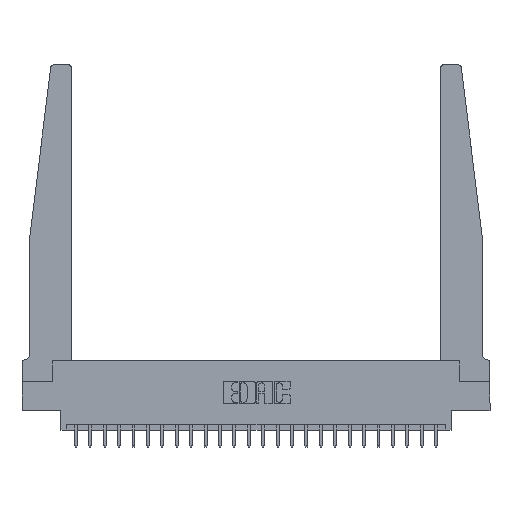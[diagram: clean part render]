
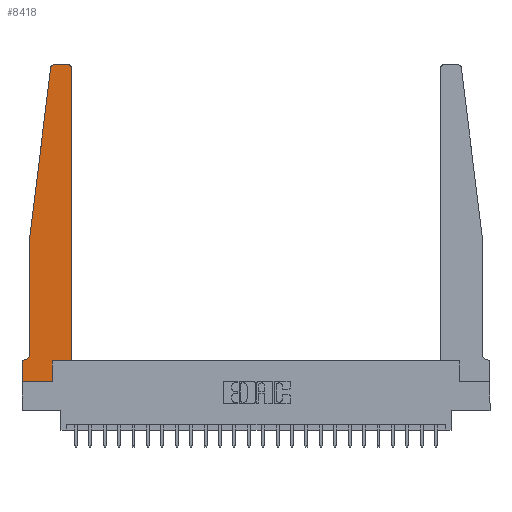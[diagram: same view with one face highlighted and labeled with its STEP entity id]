
A CAD part, top view. The second image highlights one B-rep face of the part: STEP entity #8418.
In plain terms, the highlighted planar face has unit normal (0, 0, 1).
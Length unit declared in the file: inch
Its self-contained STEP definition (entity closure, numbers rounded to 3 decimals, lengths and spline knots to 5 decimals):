
#93 = CARTESIAN_POINT ( 'NONE',  ( 0.425, 0.18, 0.37 ) ) ;
#148 = EDGE_CURVE ( 'NONE', #23735, #19029, #3038, .T. ) ;
#575 = EDGE_CURVE ( 'NONE', #8335, #3138, #4792, .T. ) ;
#618 = ORIENTED_EDGE ( 'NONE', *, *, #18903, .T. ) ;
#752 = EDGE_CURVE ( 'NONE', #6544, #5603, #20472, .T. ) ;
#990 = AXIS2_PLACEMENT_3D ( 'NONE', #11127, #23909, #12964 ) ;
#1376 = EDGE_CURVE ( 'NONE', #8189, #11717, #5085, .T. ) ;
#1635 = ORIENTED_EDGE ( 'NONE', *, *, #6350, .T. ) ;
#2336 = EDGE_CURVE ( 'NONE', #5603, #23596, #15535, .T. ) ;
#2515 = DIRECTION ( 'NONE',  ( -1., 0., 0. ) ) ;
#2861 = AXIS2_PLACEMENT_3D ( 'NONE', #17002, #5889, #18854 ) ;
#2961 = DIRECTION ( 'NONE',  ( 0., 0., 1. ) ) ;
#2983 = ORIENTED_EDGE ( 'NONE', *, *, #148, .T. ) ;
#3033 = CARTESIAN_POINT ( 'NONE',  ( 0., 0., 0.37 ) ) ;
#3038 = LINE ( 'NONE', #3033, #17319 ) ;
#3138 = VERTEX_POINT ( 'NONE', #21702 ) ;
#3180 = LINE ( 'NONE', #12296, #22329 ) ;
#3319 = ORIENTED_EDGE ( 'NONE', *, *, #752, .T. ) ;
#3325 = CARTESIAN_POINT ( 'NONE',  ( 0.2605, 0.18, 0.37 ) ) ;
#3901 = LINE ( 'NONE', #16484, #13267 ) ;
#3904 = ORIENTED_EDGE ( 'NONE', *, *, #1376, .T. ) ;
#4440 = CARTESIAN_POINT ( 'NONE',  ( 0.065, 1.25, 0.37 ) ) ;
#4792 = LINE ( 'NONE', #11908, #9237 ) ;
#5085 = LINE ( 'NONE', #21316, #9513 ) ;
#5603 = VERTEX_POINT ( 'NONE', #13830 ) ;
#5697 = VECTOR ( 'NONE', #23321, 39.37008 ) ;
#5717 = VECTOR ( 'NONE', #20847, 39.37008 ) ;
#5889 = DIRECTION ( 'NONE',  ( 0., 0., 1. ) ) ;
#6098 = FACE_OUTER_BOUND ( 'NONE', #22057, .T. ) ;
#6304 = LINE ( 'NONE', #13454, #5717 ) ;
#6350 = EDGE_CURVE ( 'NONE', #23596, #22242, #3180, .T. ) ;
#6529 = CARTESIAN_POINT ( 'NONE',  ( 0.24675, 2.72367, 0.37 ) ) ;
#6544 = VERTEX_POINT ( 'NONE', #23954 ) ;
#6770 = CIRCLE ( 'NONE', #990, 0.05 ) ;
#6865 = LINE ( 'NONE', #17923, #21574 ) ;
#7767 = VERTEX_POINT ( 'NONE', #18488 ) ;
#8189 = VERTEX_POINT ( 'NONE', #3325 ) ;
#8335 = VERTEX_POINT ( 'NONE', #9351 ) ;
#8418 = ADVANCED_FACE ( 'NONE', ( #6098 ), #11468, .T. ) ;
#8493 = ORIENTED_EDGE ( 'NONE', *, *, #13509, .T. ) ;
#8715 = DIRECTION ( 'NONE',  ( 0., -1., 0. ) ) ;
#9237 = VECTOR ( 'NONE', #2515, 39.37008 ) ;
#9351 = CARTESIAN_POINT ( 'NONE',  ( 0.015, 0.1875, 0.37 ) ) ;
#9502 = CARTESIAN_POINT ( 'NONE',  ( 0.425, 2.72, 0.37 ) ) ;
#9513 = VECTOR ( 'NONE', #19489, 39.37008 ) ;
#10317 = ORIENTED_EDGE ( 'NONE', *, *, #23913, .T. ) ;
#10349 = CARTESIAN_POINT ( 'NONE',  ( 0.425, 0.18, 0.37 ) ) ;
#10358 = DIRECTION ( 'NONE',  ( -0.122, -0.992, 0. ) ) ;
#10434 = CARTESIAN_POINT ( 'NONE',  ( 0.27653, 2.72, 0.37 ) ) ;
#10638 = CARTESIAN_POINT ( 'NONE',  ( 0., 0., 0.37 ) ) ;
#11127 = CARTESIAN_POINT ( 'NONE',  ( 0.015, 0.2375, 0.37 ) ) ;
#11468 = PLANE ( 'NONE',  #2861 ) ;
#11717 = VERTEX_POINT ( 'NONE', #93 ) ;
#11908 = CARTESIAN_POINT ( 'NONE',  ( 0.065, 0.1875, 0.37 ) ) ;
#11972 = EDGE_CURVE ( 'NONE', #11717, #16843, #14654, .T. ) ;
#12151 = ORIENTED_EDGE ( 'NONE', *, *, #575, .T. ) ;
#12212 = DIRECTION ( 'NONE',  ( 0., 1., 0. ) ) ;
#12287 = DIRECTION ( 'NONE',  ( 1., 0., 0. ) ) ;
#12296 = CARTESIAN_POINT ( 'NONE',  ( 0.065, 1.25, 0.37 ) ) ;
#12757 = AXIS2_PLACEMENT_3D ( 'NONE', #14172, #2961, #16018 ) ;
#12964 = DIRECTION ( 'NONE',  ( -1., 0., 0. ) ) ;
#13267 = VECTOR ( 'NONE', #20175, 39.37008 ) ;
#13374 = EDGE_CURVE ( 'NONE', #22242, #7767, #6865, .T. ) ;
#13454 = CARTESIAN_POINT ( 'NONE',  ( 0.2605, 0.18, 0.37 ) ) ;
#13509 = EDGE_CURVE ( 'NONE', #3138, #23735, #3901, .T. ) ;
#13830 = CARTESIAN_POINT ( 'NONE',  ( 0.27653, 2.75, 0.37 ) ) ;
#13938 = ORIENTED_EDGE ( 'NONE', *, *, #2336, .T. ) ;
#14082 = CARTESIAN_POINT ( 'NONE',  ( 0.2605, 0., 0.37 ) ) ;
#14172 = CARTESIAN_POINT ( 'NONE',  ( 0.395, 2.72, 0.37 ) ) ;
#14202 = AXIS2_PLACEMENT_3D ( 'NONE', #10434, #23232, #12287 ) ;
#14654 = LINE ( 'NONE', #10349, #18407 ) ;
#15483 = ORIENTED_EDGE ( 'NONE', *, *, #11972, .T. ) ;
#15535 = CIRCLE ( 'NONE', #14202, 0.03 ) ;
#16018 = DIRECTION ( 'NONE',  ( 1., 0., 0. ) ) ;
#16484 = CARTESIAN_POINT ( 'NONE',  ( 0., 0., 0.37 ) ) ;
#16843 = VERTEX_POINT ( 'NONE', #9502 ) ;
#17002 = CARTESIAN_POINT ( 'NONE',  ( 0., 0.1875, 0.37 ) ) ;
#17319 = VECTOR ( 'NONE', #19791, 39.37008 ) ;
#17923 = CARTESIAN_POINT ( 'NONE',  ( 0.065, 1.25, 0.37 ) ) ;
#18177 = CIRCLE ( 'NONE', #12757, 0.03 ) ;
#18407 = VECTOR ( 'NONE', #12212, 39.37008 ) ;
#18488 = CARTESIAN_POINT ( 'NONE',  ( 0.065, 0.2375, 0.37 ) ) ;
#18727 = ORIENTED_EDGE ( 'NONE', *, *, #19044, .T. ) ;
#18854 = DIRECTION ( 'NONE',  ( 1., 0., 0. ) ) ;
#18903 = EDGE_CURVE ( 'NONE', #19029, #8189, #6304, .T. ) ;
#19029 = VERTEX_POINT ( 'NONE', #14082 ) ;
#19044 = EDGE_CURVE ( 'NONE', #16843, #6544, #18177, .T. ) ;
#19489 = DIRECTION ( 'NONE',  ( 1., 0., 0. ) ) ;
#19686 = CARTESIAN_POINT ( 'NONE',  ( 0.25, 2.75, 0.37 ) ) ;
#19791 = DIRECTION ( 'NONE',  ( 1., 0., 0. ) ) ;
#20175 = DIRECTION ( 'NONE',  ( 0., -1., 0. ) ) ;
#20472 = LINE ( 'NONE', #19686, #5697 ) ;
#20847 = DIRECTION ( 'NONE',  ( 0., 1., 0. ) ) ;
#21316 = CARTESIAN_POINT ( 'NONE',  ( 0.425, 0.18, 0.37 ) ) ;
#21574 = VECTOR ( 'NONE', #8715, 39.37008 ) ;
#21702 = CARTESIAN_POINT ( 'NONE',  ( 0., 0.1875, 0.37 ) ) ;
#22057 = EDGE_LOOP ( 'NONE', ( #3319, #13938, #1635, #22476, #10317, #12151, #8493, #2983, #618, #3904, #15483, #18727 ) ) ;
#22242 = VERTEX_POINT ( 'NONE', #4440 ) ;
#22329 = VECTOR ( 'NONE', #10358, 39.37008 ) ;
#22476 = ORIENTED_EDGE ( 'NONE', *, *, #13374, .T. ) ;
#23232 = DIRECTION ( 'NONE',  ( 0., 0., 1. ) ) ;
#23321 = DIRECTION ( 'NONE',  ( -1., 0., 0. ) ) ;
#23596 = VERTEX_POINT ( 'NONE', #6529 ) ;
#23735 = VERTEX_POINT ( 'NONE', #10638 ) ;
#23909 = DIRECTION ( 'NONE',  ( 0., 0., -1. ) ) ;
#23913 = EDGE_CURVE ( 'NONE', #7767, #8335, #6770, .T. ) ;
#23954 = CARTESIAN_POINT ( 'NONE',  ( 0.395, 2.75, 0.37 ) ) ;
